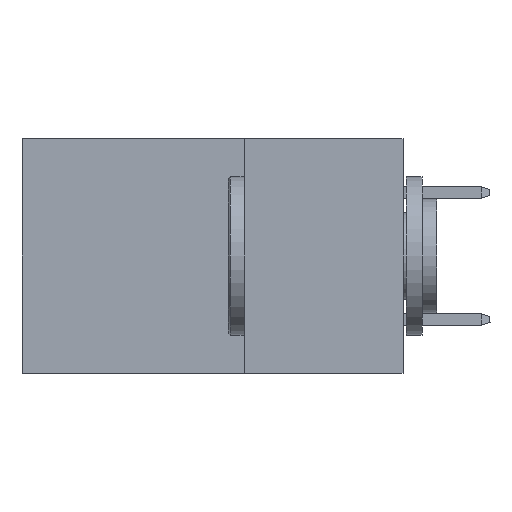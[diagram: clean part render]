
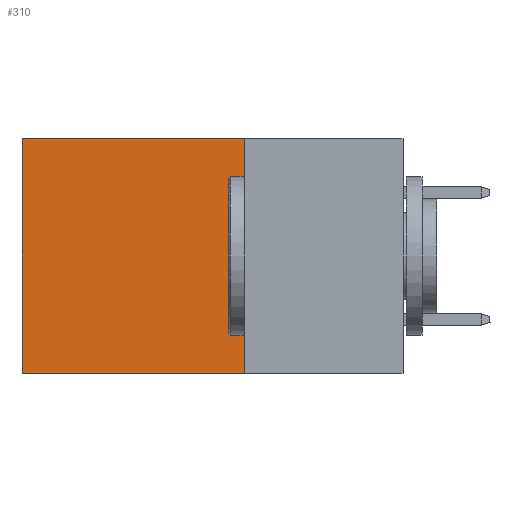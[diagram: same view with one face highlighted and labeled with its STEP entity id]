
A CAD part, left-side view. The second image highlights one B-rep face of the part: STEP entity #310.
In plain terms, the highlighted planar face has unit normal (-1, 0, 0).
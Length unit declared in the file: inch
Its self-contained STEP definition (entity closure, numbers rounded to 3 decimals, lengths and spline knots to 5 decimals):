
#227 = VECTOR ( 'NONE', #5679, 39.37008 ) ;
#310 = ADVANCED_FACE ( 'NONE', ( #11774 ), #3611, .F. ) ;
#460 = DIRECTION ( 'NONE',  ( 1., 0., 0. ) ) ;
#600 = CARTESIAN_POINT ( 'NONE',  ( 0.2875, 0.25, -0.37 ) ) ;
#713 = DIRECTION ( 'NONE',  ( 0., 0., -1. ) ) ;
#1276 = LINE ( 'NONE', #600, #7976 ) ;
#1383 = LINE ( 'NONE', #12248, #9541 ) ;
#2269 = CARTESIAN_POINT ( 'NONE',  ( 0.2875, 0.6, -0.37 ) ) ;
#2993 = DIRECTION ( 'NONE',  ( 0., 0., -1. ) ) ;
#3611 = PLANE ( 'NONE',  #9198 ) ;
#3888 = VERTEX_POINT ( 'NONE', #12327 ) ;
#4368 = ORIENTED_EDGE ( 'NONE', *, *, #8543, .F. ) ;
#4715 = VERTEX_POINT ( 'NONE', #8751 ) ;
#5679 = DIRECTION ( 'NONE',  ( 0., 1., 0. ) ) ;
#5700 = ORIENTED_EDGE ( 'NONE', *, *, #10936, .T. ) ;
#5952 = VECTOR ( 'NONE', #2993, 39.37008 ) ;
#7170 = VERTEX_POINT ( 'NONE', #8110 ) ;
#7961 = DIRECTION ( 'NONE',  ( 0., 1., 0. ) ) ;
#7976 = VECTOR ( 'NONE', #7961, 39.37008 ) ;
#8110 = CARTESIAN_POINT ( 'NONE',  ( 0.2875, 0.25, 0. ) ) ;
#8543 = EDGE_CURVE ( 'NONE', #7170, #3888, #1383, .T. ) ;
#8751 = CARTESIAN_POINT ( 'NONE',  ( 0.2875, 0.6, 0. ) ) ;
#8989 = LINE ( 'NONE', #12218, #227 ) ;
#9091 = DIRECTION ( 'NONE',  ( 0., 0., -1. ) ) ;
#9198 = AXIS2_PLACEMENT_3D ( 'NONE', #13540, #460, #713 ) ;
#9541 = VECTOR ( 'NONE', #9091, 39.37008 ) ;
#10313 = EDGE_CURVE ( 'NONE', #3888, #11400, #1276, .T. ) ;
#10936 = EDGE_CURVE ( 'NONE', #4715, #11400, #11301, .T. ) ;
#11301 = LINE ( 'NONE', #13511, #5952 ) ;
#11400 = VERTEX_POINT ( 'NONE', #2269 ) ;
#11774 = FACE_OUTER_BOUND ( 'NONE', #13721, .T. ) ;
#12173 = ORIENTED_EDGE ( 'NONE', *, *, #14104, .T. ) ;
#12218 = CARTESIAN_POINT ( 'NONE',  ( 0.2875, 0.25, 0. ) ) ;
#12248 = CARTESIAN_POINT ( 'NONE',  ( 0.2875, 0.25, 0. ) ) ;
#12327 = CARTESIAN_POINT ( 'NONE',  ( 0.2875, 0.25, -0.37 ) ) ;
#13508 = ORIENTED_EDGE ( 'NONE', *, *, #10313, .F. ) ;
#13511 = CARTESIAN_POINT ( 'NONE',  ( 0.2875, 0.6, 0. ) ) ;
#13540 = CARTESIAN_POINT ( 'NONE',  ( 0.2875, 0.25, 0. ) ) ;
#13721 = EDGE_LOOP ( 'NONE', ( #5700, #13508, #4368, #12173 ) ) ;
#14104 = EDGE_CURVE ( 'NONE', #7170, #4715, #8989, .T. ) ;
